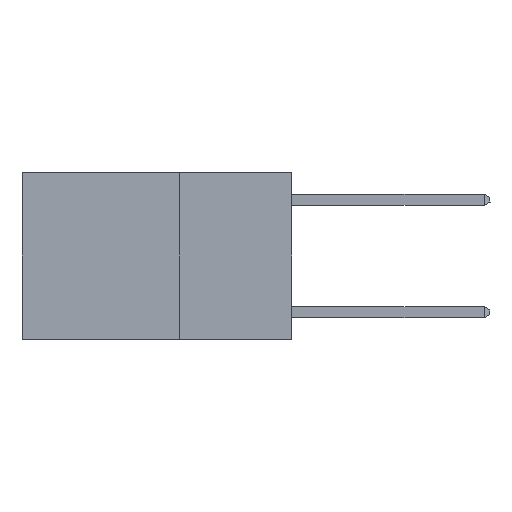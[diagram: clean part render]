
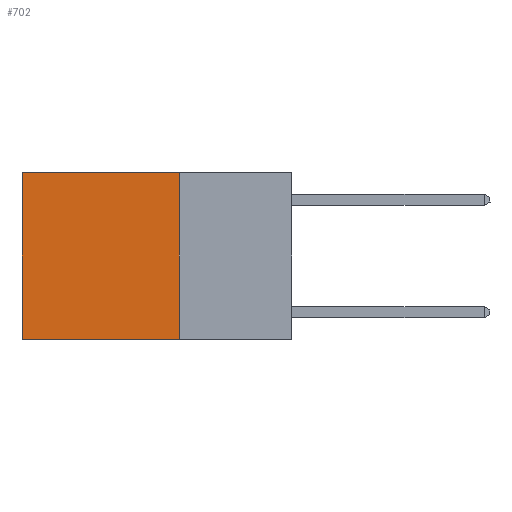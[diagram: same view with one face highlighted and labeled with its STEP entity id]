
A CAD part, left-side view. The second image highlights one B-rep face of the part: STEP entity #702.
In plain terms, the highlighted planar face has unit normal (-1, 0, 0).
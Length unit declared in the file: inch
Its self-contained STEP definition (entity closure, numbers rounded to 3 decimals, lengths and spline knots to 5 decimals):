
#38 = CARTESIAN_POINT ( 'NONE',  ( 0.2625, 0.6, -0.37 ) ) ;
#648 = CARTESIAN_POINT ( 'NONE',  ( 0.2625, 0.25, 0. ) ) ;
#702 = ADVANCED_FACE ( 'NONE', ( #5366 ), #7791, .F. ) ;
#862 = DIRECTION ( 'NONE',  ( 0., 1., 0. ) ) ;
#1586 = DIRECTION ( 'NONE',  ( 0., 0., -1. ) ) ;
#1962 = VERTEX_POINT ( 'NONE', #7678 ) ;
#2499 = VERTEX_POINT ( 'NONE', #2949 ) ;
#2949 = CARTESIAN_POINT ( 'NONE',  ( 0.2625, 0.25, -0.37 ) ) ;
#3237 = ORIENTED_EDGE ( 'NONE', *, *, #6845, .T. ) ;
#3274 = ORIENTED_EDGE ( 'NONE', *, *, #6531, .T. ) ;
#3319 = ORIENTED_EDGE ( 'NONE', *, *, #7965, .F. ) ;
#3390 = ORIENTED_EDGE ( 'NONE', *, *, #7396, .F. ) ;
#3418 = CARTESIAN_POINT ( 'NONE',  ( 0.2625, 0.25, 0. ) ) ;
#3795 = VECTOR ( 'NONE', #862, 39.37008 ) ;
#4053 = DIRECTION ( 'NONE',  ( 0., 0., -1. ) ) ;
#4153 = DIRECTION ( 'NONE',  ( 0., 0., -1. ) ) ;
#4803 = EDGE_LOOP ( 'NONE', ( #3237, #3319, #3390, #3274 ) ) ;
#5023 = VECTOR ( 'NONE', #4153, 39.37008 ) ;
#5035 = VERTEX_POINT ( 'NONE', #3418 ) ;
#5366 = FACE_OUTER_BOUND ( 'NONE', #4803, .T. ) ;
#5384 = VECTOR ( 'NONE', #1586, 39.37008 ) ;
#6519 = CARTESIAN_POINT ( 'NONE',  ( 0.2625, 0.6, 0. ) ) ;
#6531 = EDGE_CURVE ( 'NONE', #5035, #1962, #9362, .T. ) ;
#6845 = EDGE_CURVE ( 'NONE', #1962, #8018, #7198, .T. ) ;
#7061 = CARTESIAN_POINT ( 'NONE',  ( 0.2625, 0.25, 0. ) ) ;
#7198 = LINE ( 'NONE', #6519, #5023 ) ;
#7342 = VECTOR ( 'NONE', #10071, 39.37008 ) ;
#7396 = EDGE_CURVE ( 'NONE', #5035, #2499, #7578, .T. ) ;
#7578 = LINE ( 'NONE', #648, #5384 ) ;
#7678 = CARTESIAN_POINT ( 'NONE',  ( 0.2625, 0.6, 0. ) ) ;
#7791 = PLANE ( 'NONE',  #7919 ) ;
#7863 = DIRECTION ( 'NONE',  ( 1., 0., 0. ) ) ;
#7919 = AXIS2_PLACEMENT_3D ( 'NONE', #8193, #7863, #4053 ) ;
#7965 = EDGE_CURVE ( 'NONE', #2499, #8018, #9997, .T. ) ;
#8018 = VERTEX_POINT ( 'NONE', #38 ) ;
#8193 = CARTESIAN_POINT ( 'NONE',  ( 0.2625, 0.25, 0. ) ) ;
#9362 = LINE ( 'NONE', #7061, #7342 ) ;
#9997 = LINE ( 'NONE', #10354, #3795 ) ;
#10071 = DIRECTION ( 'NONE',  ( 0., 1., 0. ) ) ;
#10354 = CARTESIAN_POINT ( 'NONE',  ( 0.2625, 0.25, -0.37 ) ) ;
